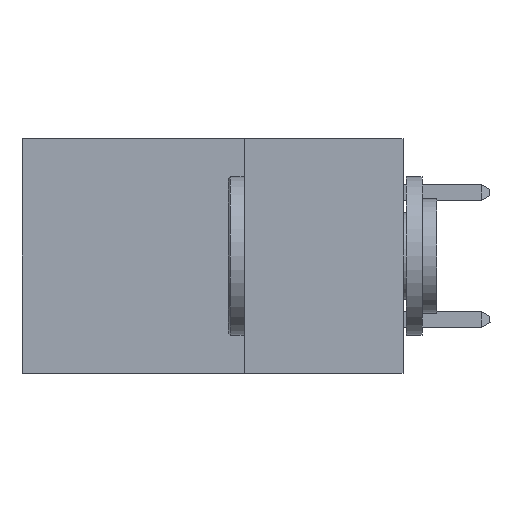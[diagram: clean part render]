
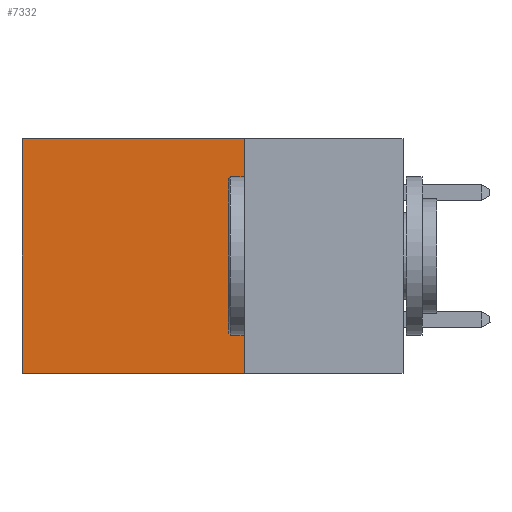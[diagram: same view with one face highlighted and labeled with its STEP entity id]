
A CAD part, left-side view. The second image highlights one B-rep face of the part: STEP entity #7332.
In plain terms, the highlighted planar face has unit normal (-1, 0, 0).
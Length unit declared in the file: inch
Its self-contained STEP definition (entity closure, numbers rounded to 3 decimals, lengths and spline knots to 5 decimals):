
#379 = CARTESIAN_POINT ( 'NONE',  ( 0.2875, 0.6, -0.37 ) ) ;
#674 = EDGE_CURVE ( 'NONE', #2979, #10090, #16896, .T. ) ;
#819 = VERTEX_POINT ( 'NONE', #379 ) ;
#978 = VECTOR ( 'NONE', #12433, 39.37008 ) ;
#2687 = VECTOR ( 'NONE', #5411, 39.37008 ) ;
#2979 = VERTEX_POINT ( 'NONE', #21608 ) ;
#3898 = VECTOR ( 'NONE', #20826, 39.37008 ) ;
#4900 = CARTESIAN_POINT ( 'NONE',  ( 0.2875, 0.25, 0. ) ) ;
#5140 = CARTESIAN_POINT ( 'NONE',  ( 0.2875, 0.25, 0. ) ) ;
#5411 = DIRECTION ( 'NONE',  ( 0., 1., 0. ) ) ;
#6201 = AXIS2_PLACEMENT_3D ( 'NONE', #20580, #9937, #22331 ) ;
#7332 = ADVANCED_FACE ( 'NONE', ( #20811 ), #16997, .F. ) ;
#7606 = EDGE_CURVE ( 'NONE', #16211, #819, #15230, .T. ) ;
#9433 = EDGE_CURVE ( 'NONE', #10090, #819, #20105, .T. ) ;
#9459 = ORIENTED_EDGE ( 'NONE', *, *, #21320, .F. ) ;
#9937 = DIRECTION ( 'NONE',  ( 1., 0., 0. ) ) ;
#10090 = VERTEX_POINT ( 'NONE', #21448 ) ;
#10634 = CARTESIAN_POINT ( 'NONE',  ( 0.2875, 0.25, -0.37 ) ) ;
#12433 = DIRECTION ( 'NONE',  ( 0., 1., 0. ) ) ;
#12750 = EDGE_LOOP ( 'NONE', ( #21084, #18439, #9459, #12848 ) ) ;
#12848 = ORIENTED_EDGE ( 'NONE', *, *, #674, .T. ) ;
#15230 = LINE ( 'NONE', #10634, #978 ) ;
#16211 = VERTEX_POINT ( 'NONE', #22461 ) ;
#16896 = LINE ( 'NONE', #5140, #2687 ) ;
#16997 = PLANE ( 'NONE',  #6201 ) ;
#17460 = CARTESIAN_POINT ( 'NONE',  ( 0.2875, 0.6, 0. ) ) ;
#18095 = LINE ( 'NONE', #4900, #3898 ) ;
#18439 = ORIENTED_EDGE ( 'NONE', *, *, #7606, .F. ) ;
#20105 = LINE ( 'NONE', #17460, #20637 ) ;
#20580 = CARTESIAN_POINT ( 'NONE',  ( 0.2875, 0.25, 0. ) ) ;
#20637 = VECTOR ( 'NONE', #21017, 39.37008 ) ;
#20811 = FACE_OUTER_BOUND ( 'NONE', #12750, .T. ) ;
#20826 = DIRECTION ( 'NONE',  ( 0., 0., -1. ) ) ;
#21017 = DIRECTION ( 'NONE',  ( 0., 0., -1. ) ) ;
#21084 = ORIENTED_EDGE ( 'NONE', *, *, #9433, .T. ) ;
#21320 = EDGE_CURVE ( 'NONE', #2979, #16211, #18095, .T. ) ;
#21448 = CARTESIAN_POINT ( 'NONE',  ( 0.2875, 0.6, 0. ) ) ;
#21608 = CARTESIAN_POINT ( 'NONE',  ( 0.2875, 0.25, 0. ) ) ;
#22331 = DIRECTION ( 'NONE',  ( 0., 0., -1. ) ) ;
#22461 = CARTESIAN_POINT ( 'NONE',  ( 0.2875, 0.25, -0.37 ) ) ;
